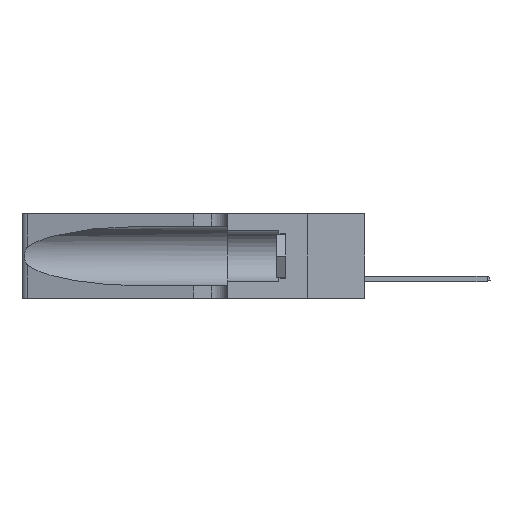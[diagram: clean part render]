
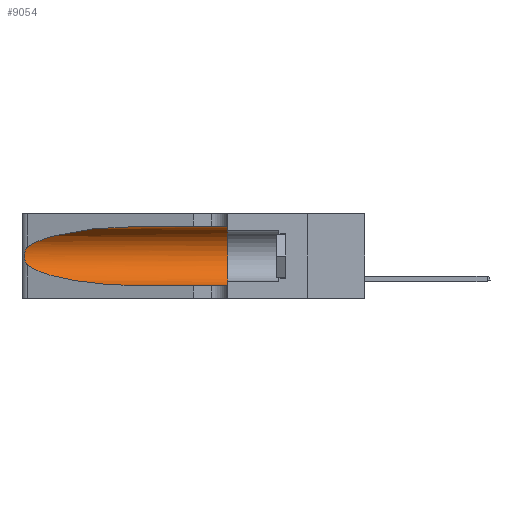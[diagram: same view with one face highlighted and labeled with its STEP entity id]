
A CAD part, left-side view. The second image highlights one B-rep face of the part: STEP entity #9054.
In plain terms, the highlighted cylindrical face has radius 3.308 mm (diameter 6.617 mm), a partial arc.
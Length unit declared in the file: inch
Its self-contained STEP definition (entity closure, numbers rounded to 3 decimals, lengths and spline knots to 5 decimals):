
#38 = CARTESIAN_POINT ( 'NONE',  ( 0.26017, 1.23833, 0.17102 ) ) ;
#164 = CARTESIAN_POINT ( 'NONE',  ( 0.1305, 0.72297, 0.31525 ) ) ;
#390 = DIRECTION ( 'NONE',  ( 0., -1., 0. ) ) ;
#729 = EDGE_CURVE ( 'NONE', #11029, #20309, #5360, .T. ) ;
#878 = ORIENTED_EDGE ( 'NONE', *, *, #22854, .T. ) ;
#1207 = AXIS2_PLACEMENT_3D ( 'NONE', #16099, #23911, #20457 ) ;
#1698 = ORIENTED_EDGE ( 'NONE', *, *, #729, .T. ) ;
#1703 = CARTESIAN_POINT ( 'NONE',  ( 0.26018, 1.23835, 0.19895 ) ) ;
#2064 = EDGE_CURVE ( 'NONE', #5413, #20309, #18068, .T. ) ;
#2158 = CARTESIAN_POINT ( 'NONE',  ( 0.25487, 1.22718, 0.22369 ) ) ;
#2474 = CARTESIAN_POINT ( 'NONE',  ( 0.1305, 0.35, 0.185 ) ) ;
#3704 = VERTEX_POINT ( 'NONE', #6559 ) ;
#3806 = CARTESIAN_POINT ( 'NONE',  ( 0.25639, 1.23184, 0.21858 ) ) ;
#3968 = CARTESIAN_POINT ( 'NONE',  ( 0.25487, 1.22718, 0.22369 ) ) ;
#4011 = EDGE_CURVE ( 'NONE', #10032, #5413, #24143, .T. ) ;
#4902 = CARTESIAN_POINT ( 'NONE',  ( 0.1305, 0.35, 0.31525 ) ) ;
#5223 = CARTESIAN_POINT ( 'NONE',  ( 0.18966, 0.96281, 0.05475 ) ) ;
#5360 = LINE ( 'NONE', #12341, #21558 ) ;
#5413 = VERTEX_POINT ( 'NONE', #4902 ) ;
#5687 = B_SPLINE_CURVE_WITH_KNOTS ( 'NONE', 3,
 ( #3968, #5967, #3806, #18005, #23865, #1703, #23691, #19908, #38, #15970, #11890, #21892, #21647, #11640 ),
 .UNSPECIFIED., .F., .F.,
 ( 4, 2, 2, 2, 2, 2, 4 ),
 ( 0., 0.00027, 0.00053, 0.00107, 0.0016, 0.00187, 0.00214 ),
 .UNSPECIFIED. ) ;
#5967 = CARTESIAN_POINT ( 'NONE',  ( 0.25555, 1.22994, 0.2215 ) ) ;
#6087 = CARTESIAN_POINT ( 'NONE',  ( 0.18966, 0.96281, 0.31525 ) ) ;
#6559 = CARTESIAN_POINT ( 'NONE',  ( 0.25487, 1.22718, 0.14631 ) ) ;
#7162 = CARTESIAN_POINT ( 'NONE',  ( 0.1305, 0.72297, 0.05475 ) ) ;
#8244 = FACE_OUTER_BOUND ( 'NONE', #8561, .T. ) ;
#8259 = CARTESIAN_POINT ( 'NONE',  ( 0.1305, 0.72297, 0.05475 ) ) ;
#8561 = EDGE_LOOP ( 'NONE', ( #21540, #12841, #878, #1698, #19689, #9175 ) ) ;
#9054 = ADVANCED_FACE ( 'NONE', ( #8244 ), #14759, .F. ) ;
#9097 = DIRECTION ( 'NONE',  ( 0., 1., 0. ) ) ;
#9103 = DIRECTION ( 'NONE',  ( 0., -1., 0. ) ) ;
#9175 = ORIENTED_EDGE ( 'NONE', *, *, #4011, .F. ) ;
#9983 = AXIS2_PLACEMENT_3D ( 'NONE', #2474, #9097, #17011 ) ;
#10032 = VERTEX_POINT ( 'NONE', #18944 ) ;
#11029 = VERTEX_POINT ( 'NONE', #8259 ) ;
#11160 = CARTESIAN_POINT ( 'NONE',  ( 0.25487, 1.22718, 0.14631 ) ) ;
#11640 = CARTESIAN_POINT ( 'NONE',  ( 0.25487, 1.22718, 0.14631 ) ) ;
#11890 = CARTESIAN_POINT ( 'NONE',  ( 0.25789, 1.23486, 0.15765 ) ) ;
#12341 = CARTESIAN_POINT ( 'NONE',  ( 0.1305, 1.61858, 0.05475 ) ) ;
#12349 = VECTOR ( 'NONE', #9103, 39.37008 ) ;
#12841 = ORIENTED_EDGE ( 'NONE', *, *, #24641, .T. ) ;
#13344 =( BOUNDED_CURVE ( )  B_SPLINE_CURVE ( 3, ( #11160, #22797, #5223, #7162 ),
 .UNSPECIFIED., .F., .F. ) 
 B_SPLINE_CURVE_WITH_KNOTS ( ( 4, 4 ),
 ( 3.44316, 4.71239 ),
 .UNSPECIFIED. ) 
 CURVE ( )  GEOMETRIC_REPRESENTATION_ITEM ( )  RATIONAL_B_SPLINE_CURVE ( ( 1., 0.87, 0.87, 1. ) ) 
 REPRESENTATION_ITEM ( '' )  );
#14759 = CYLINDRICAL_SURFACE ( 'NONE', #1207, 0.13025 ) ;
#15970 = CARTESIAN_POINT ( 'NONE',  ( 0.25856, 1.23593, 0.16098 ) ) ;
#16099 = CARTESIAN_POINT ( 'NONE',  ( 0.1305, 1.61858, 0.185 ) ) ;
#17011 = DIRECTION ( 'NONE',  ( 0., 0., 1. ) ) ;
#17884 = EDGE_CURVE ( 'NONE', #10032, #21404, #18002, .T. ) ;
#18002 =( BOUNDED_CURVE ( )  B_SPLINE_CURVE ( 3, ( #164, #6087, #18723, #2158 ),
 .UNSPECIFIED., .F., .T. ) 
 B_SPLINE_CURVE_WITH_KNOTS ( ( 4, 4 ),
 ( 1.5708, 2.84003 ),
 .UNSPECIFIED. ) 
 CURVE ( )  GEOMETRIC_REPRESENTATION_ITEM ( )  RATIONAL_B_SPLINE_CURVE ( ( 1., 0.87, 0.87, 1. ) ) 
 REPRESENTATION_ITEM ( '' )  );
#18005 = CARTESIAN_POINT ( 'NONE',  ( 0.25787, 1.23484, 0.2124 ) ) ;
#18068 = CIRCLE ( 'NONE', #9983, 0.13025 ) ;
#18356 = CARTESIAN_POINT ( 'NONE',  ( 0.1305, 0.35, 0.05475 ) ) ;
#18723 = CARTESIAN_POINT ( 'NONE',  ( 0.2373, 1.15595, 0.28018 ) ) ;
#18944 = CARTESIAN_POINT ( 'NONE',  ( 0.1305, 0.72297, 0.31525 ) ) ;
#19689 = ORIENTED_EDGE ( 'NONE', *, *, #2064, .F. ) ;
#19908 = CARTESIAN_POINT ( 'NONE',  ( 0.26075, 1.23896, 0.178 ) ) ;
#20309 = VERTEX_POINT ( 'NONE', #18356 ) ;
#20457 = DIRECTION ( 'NONE',  ( 0., 0., -1. ) ) ;
#21404 = VERTEX_POINT ( 'NONE', #23444 ) ;
#21540 = ORIENTED_EDGE ( 'NONE', *, *, #17884, .T. ) ;
#21558 = VECTOR ( 'NONE', #390, 39.37008 ) ;
#21647 = CARTESIAN_POINT ( 'NONE',  ( 0.25555, 1.22993, 0.14849 ) ) ;
#21892 = CARTESIAN_POINT ( 'NONE',  ( 0.25639, 1.23186, 0.15144 ) ) ;
#22797 = CARTESIAN_POINT ( 'NONE',  ( 0.2373, 1.15595, 0.08982 ) ) ;
#22854 = EDGE_CURVE ( 'NONE', #3704, #11029, #13344, .T. ) ;
#23444 = CARTESIAN_POINT ( 'NONE',  ( 0.25487, 1.22718, 0.22369 ) ) ;
#23691 = CARTESIAN_POINT ( 'NONE',  ( 0.26075, 1.23896, 0.19203 ) ) ;
#23865 = CARTESIAN_POINT ( 'NONE',  ( 0.25854, 1.2359, 0.20912 ) ) ;
#23911 = DIRECTION ( 'NONE',  ( 0., -1., 0. ) ) ;
#24143 = LINE ( 'NONE', #25158, #12349 ) ;
#24641 = EDGE_CURVE ( 'NONE', #21404, #3704, #5687, .T. ) ;
#25158 = CARTESIAN_POINT ( 'NONE',  ( 0.1305, 1.61858, 0.31525 ) ) ;
